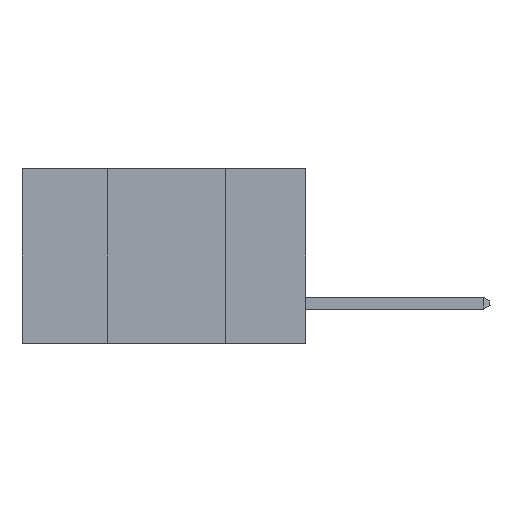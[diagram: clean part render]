
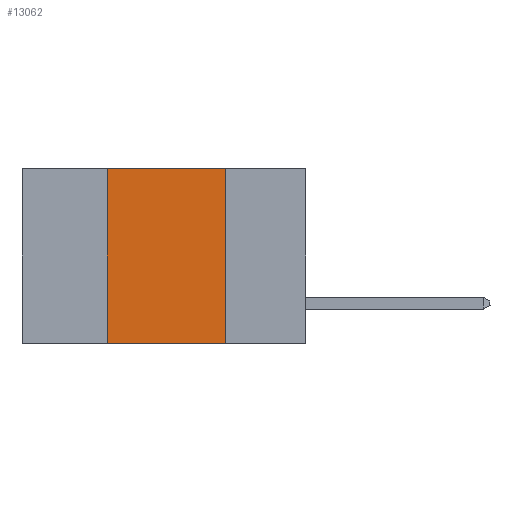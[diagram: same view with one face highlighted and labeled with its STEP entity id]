
A CAD part, left-side view. The second image highlights one B-rep face of the part: STEP entity #13062.
In plain terms, the highlighted planar face has unit normal (-1, 0, 0).
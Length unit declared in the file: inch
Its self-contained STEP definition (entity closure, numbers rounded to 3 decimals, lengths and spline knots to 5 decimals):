
#202 = DIRECTION ( 'NONE',  ( 0., 0., 1. ) ) ;
#249 = CARTESIAN_POINT ( 'NONE',  ( 0., 0.42, 0. ) ) ;
#989 = LINE ( 'NONE', #6156, #11431 ) ;
#1012 = VERTEX_POINT ( 'NONE', #12514 ) ;
#1498 = CARTESIAN_POINT ( 'NONE',  ( 0., 0.17, 0. ) ) ;
#1773 = VECTOR ( 'NONE', #5917, 39.37008 ) ;
#2479 = EDGE_CURVE ( 'NONE', #3456, #7290, #5534, .T. ) ;
#2817 = AXIS2_PLACEMENT_3D ( 'NONE', #8446, #5297, #12659 ) ;
#2913 = ORIENTED_EDGE ( 'NONE', *, *, #11217, .F. ) ;
#3011 = EDGE_CURVE ( 'NONE', #1012, #7290, #7987, .T. ) ;
#3333 = ORIENTED_EDGE ( 'NONE', *, *, #3011, .F. ) ;
#3456 = VERTEX_POINT ( 'NONE', #7729 ) ;
#3901 = LINE ( 'NONE', #249, #5043 ) ;
#4284 = PLANE ( 'NONE',  #2817 ) ;
#4307 = CARTESIAN_POINT ( 'NONE',  ( 0., 0.42, 0. ) ) ;
#5043 = VECTOR ( 'NONE', #202, 39.37008 ) ;
#5258 = CARTESIAN_POINT ( 'NONE',  ( 0., 0.17, -0.37 ) ) ;
#5297 = DIRECTION ( 'NONE',  ( 1., 0., 0. ) ) ;
#5534 = LINE ( 'NONE', #11213, #1773 ) ;
#5586 = DIRECTION ( 'NONE',  ( 0., 0., -1. ) ) ;
#5917 = DIRECTION ( 'NONE',  ( 0., -1., 0. ) ) ;
#6156 = CARTESIAN_POINT ( 'NONE',  ( 0., 0.6, 0. ) ) ;
#6712 = ORIENTED_EDGE ( 'NONE', *, *, #8760, .F. ) ;
#6885 = EDGE_LOOP ( 'NONE', ( #3333, #6712, #2913, #12947 ) ) ;
#7169 = VECTOR ( 'NONE', #5586, 39.37008 ) ;
#7290 = VERTEX_POINT ( 'NONE', #5258 ) ;
#7729 = CARTESIAN_POINT ( 'NONE',  ( 0., 0.42, -0.37 ) ) ;
#7987 = LINE ( 'NONE', #1498, #7169 ) ;
#8446 = CARTESIAN_POINT ( 'NONE',  ( 0., 0.6, 0. ) ) ;
#8760 = EDGE_CURVE ( 'NONE', #10021, #1012, #989, .T. ) ;
#9477 = DIRECTION ( 'NONE',  ( 0., -1., 0. ) ) ;
#9580 = FACE_OUTER_BOUND ( 'NONE', #6885, .T. ) ;
#10021 = VERTEX_POINT ( 'NONE', #4307 ) ;
#11213 = CARTESIAN_POINT ( 'NONE',  ( 0., 0.6, -0.37 ) ) ;
#11217 = EDGE_CURVE ( 'NONE', #3456, #10021, #3901, .T. ) ;
#11431 = VECTOR ( 'NONE', #9477, 39.37008 ) ;
#12514 = CARTESIAN_POINT ( 'NONE',  ( 0., 0.17, 0. ) ) ;
#12659 = DIRECTION ( 'NONE',  ( 0., 0., -1. ) ) ;
#12947 = ORIENTED_EDGE ( 'NONE', *, *, #2479, .T. ) ;
#13062 = ADVANCED_FACE ( 'NONE', ( #9580 ), #4284, .F. ) ;
